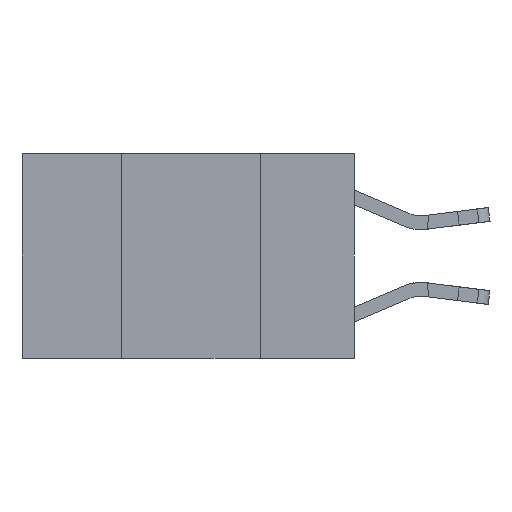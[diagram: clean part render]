
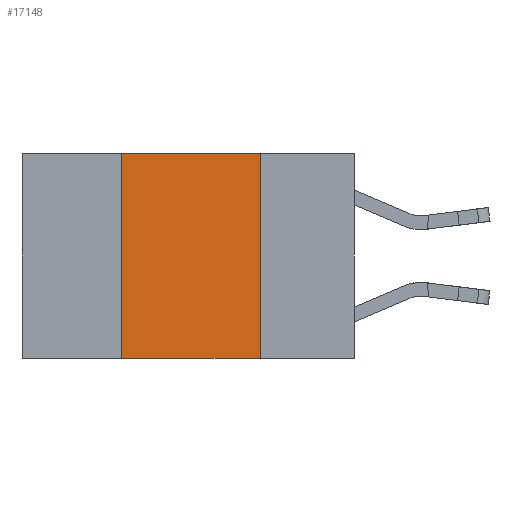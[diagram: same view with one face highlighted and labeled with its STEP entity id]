
A CAD part, left-side view. The second image highlights one B-rep face of the part: STEP entity #17148.
In plain terms, the highlighted planar face has unit normal (-1, 0, 0).
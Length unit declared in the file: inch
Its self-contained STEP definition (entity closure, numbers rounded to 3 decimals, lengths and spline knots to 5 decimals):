
#244 = CARTESIAN_POINT ( 'NONE',  ( 0., 0.17, -0.37 ) ) ;
#810 = DIRECTION ( 'NONE',  ( 0., 0., -1. ) ) ;
#1513 = CARTESIAN_POINT ( 'NONE',  ( 0., 0.42, 0. ) ) ;
#1599 = ORIENTED_EDGE ( 'NONE', *, *, #7887, .F. ) ;
#2589 = EDGE_CURVE ( 'NONE', #20099, #4596, #7242, .T. ) ;
#2620 = DIRECTION ( 'NONE',  ( 0., -1., 0. ) ) ;
#3296 = VERTEX_POINT ( 'NONE', #6537 ) ;
#3755 = DIRECTION ( 'NONE',  ( 0., -1., 0. ) ) ;
#4308 = LINE ( 'NONE', #17212, #7510 ) ;
#4596 = VERTEX_POINT ( 'NONE', #1513 ) ;
#4858 = EDGE_LOOP ( 'NONE', ( #1599, #17427, #19556, #19443 ) ) ;
#6537 = CARTESIAN_POINT ( 'NONE',  ( 0., 0.17, 0. ) ) ;
#7242 = LINE ( 'NONE', #15491, #20052 ) ;
#7510 = VECTOR ( 'NONE', #2620, 39.37008 ) ;
#7887 = EDGE_CURVE ( 'NONE', #3296, #18502, #9126, .T. ) ;
#7905 = CARTESIAN_POINT ( 'NONE',  ( 0., 0.6, 0. ) ) ;
#9015 = CARTESIAN_POINT ( 'NONE',  ( 0., 0.42, -0.37 ) ) ;
#9126 = LINE ( 'NONE', #12234, #17882 ) ;
#9958 = FACE_OUTER_BOUND ( 'NONE', #4858, .T. ) ;
#10374 = LINE ( 'NONE', #20171, #10437 ) ;
#10437 = VECTOR ( 'NONE', #3755, 39.37008 ) ;
#12195 = DIRECTION ( 'NONE',  ( 0., 0., 1. ) ) ;
#12234 = CARTESIAN_POINT ( 'NONE',  ( 0., 0.17, 0. ) ) ;
#13262 = DIRECTION ( 'NONE',  ( 0., 0., -1. ) ) ;
#14441 = PLANE ( 'NONE',  #18445 ) ;
#15491 = CARTESIAN_POINT ( 'NONE',  ( 0., 0.42, 0. ) ) ;
#16530 = DIRECTION ( 'NONE',  ( 1., 0., 0. ) ) ;
#16654 = EDGE_CURVE ( 'NONE', #4596, #3296, #4308, .T. ) ;
#17148 = ADVANCED_FACE ( 'NONE', ( #9958 ), #14441, .F. ) ;
#17212 = CARTESIAN_POINT ( 'NONE',  ( 0., 0.6, 0. ) ) ;
#17427 = ORIENTED_EDGE ( 'NONE', *, *, #16654, .F. ) ;
#17882 = VECTOR ( 'NONE', #810, 39.37008 ) ;
#18445 = AXIS2_PLACEMENT_3D ( 'NONE', #7905, #16530, #13262 ) ;
#18502 = VERTEX_POINT ( 'NONE', #244 ) ;
#18615 = EDGE_CURVE ( 'NONE', #20099, #18502, #10374, .T. ) ;
#19443 = ORIENTED_EDGE ( 'NONE', *, *, #18615, .T. ) ;
#19556 = ORIENTED_EDGE ( 'NONE', *, *, #2589, .F. ) ;
#20052 = VECTOR ( 'NONE', #12195, 39.37008 ) ;
#20099 = VERTEX_POINT ( 'NONE', #9015 ) ;
#20171 = CARTESIAN_POINT ( 'NONE',  ( 0., 0.6, -0.37 ) ) ;
